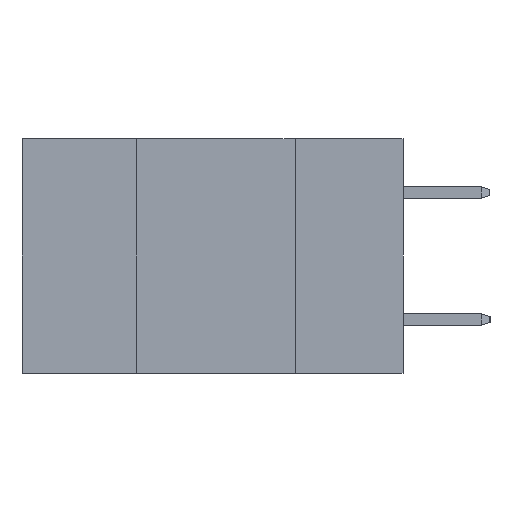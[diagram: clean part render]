
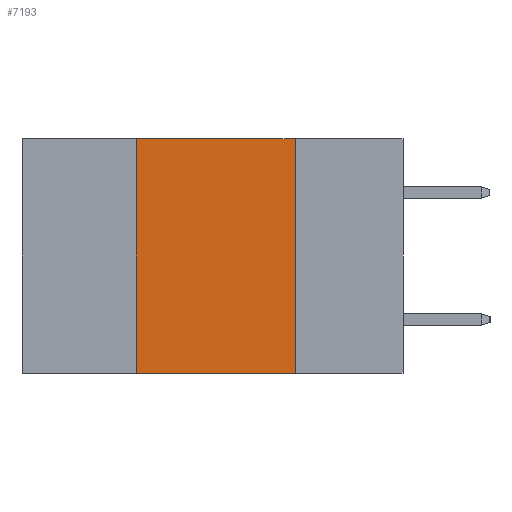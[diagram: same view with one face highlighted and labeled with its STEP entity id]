
A CAD part, left-side view. The second image highlights one B-rep face of the part: STEP entity #7193.
In plain terms, the highlighted planar face has unit normal (-1, 0, 0).
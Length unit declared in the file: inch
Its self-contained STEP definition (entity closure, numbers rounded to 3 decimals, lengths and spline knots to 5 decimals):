
#375 = CARTESIAN_POINT ( 'NONE',  ( 0., 0.42, 0. ) ) ;
#412 = CARTESIAN_POINT ( 'NONE',  ( 0., 0.6, 0. ) ) ;
#501 = EDGE_LOOP ( 'NONE', ( #10913, #5267, #13035, #7974 ) ) ;
#1068 = LINE ( 'NONE', #7234, #1835 ) ;
#1313 = CARTESIAN_POINT ( 'NONE',  ( 0., 0.42, 0. ) ) ;
#1835 = VECTOR ( 'NONE', #4190, 39.37008 ) ;
#2723 = VERTEX_POINT ( 'NONE', #14095 ) ;
#3085 = DIRECTION ( 'NONE',  ( 0., 0., -1. ) ) ;
#3303 = VERTEX_POINT ( 'NONE', #8169 ) ;
#3322 = VERTEX_POINT ( 'NONE', #375 ) ;
#4190 = DIRECTION ( 'NONE',  ( 0., 0., -1. ) ) ;
#4582 = LINE ( 'NONE', #5906, #6327 ) ;
#5114 = AXIS2_PLACEMENT_3D ( 'NONE', #10607, #6143, #3085 ) ;
#5267 = ORIENTED_EDGE ( 'NONE', *, *, #6508, .F. ) ;
#5906 = CARTESIAN_POINT ( 'NONE',  ( 0., 0.6, -0.37 ) ) ;
#6143 = DIRECTION ( 'NONE',  ( 1., 0., 0. ) ) ;
#6327 = VECTOR ( 'NONE', #15451, 39.37008 ) ;
#6508 = EDGE_CURVE ( 'NONE', #3322, #11072, #12897, .T. ) ;
#7193 = ADVANCED_FACE ( 'NONE', ( #19966 ), #18652, .F. ) ;
#7234 = CARTESIAN_POINT ( 'NONE',  ( 0., 0.17, 0. ) ) ;
#7974 = ORIENTED_EDGE ( 'NONE', *, *, #15948, .T. ) ;
#8125 = VECTOR ( 'NONE', #17045, 39.37008 ) ;
#8169 = CARTESIAN_POINT ( 'NONE',  ( 0., 0.17, -0.37 ) ) ;
#9642 = DIRECTION ( 'NONE',  ( 0., -1., 0. ) ) ;
#10607 = CARTESIAN_POINT ( 'NONE',  ( 0., 0.6, 0. ) ) ;
#10913 = ORIENTED_EDGE ( 'NONE', *, *, #19184, .F. ) ;
#11072 = VERTEX_POINT ( 'NONE', #16658 ) ;
#11674 = EDGE_CURVE ( 'NONE', #2723, #3322, #19893, .T. ) ;
#12897 = LINE ( 'NONE', #412, #13851 ) ;
#13035 = ORIENTED_EDGE ( 'NONE', *, *, #11674, .F. ) ;
#13851 = VECTOR ( 'NONE', #9642, 39.37008 ) ;
#14095 = CARTESIAN_POINT ( 'NONE',  ( 0., 0.42, -0.37 ) ) ;
#15451 = DIRECTION ( 'NONE',  ( 0., -1., 0. ) ) ;
#15948 = EDGE_CURVE ( 'NONE', #2723, #3303, #4582, .T. ) ;
#16658 = CARTESIAN_POINT ( 'NONE',  ( 0., 0.17, 0. ) ) ;
#17045 = DIRECTION ( 'NONE',  ( 0., 0., 1. ) ) ;
#18652 = PLANE ( 'NONE',  #5114 ) ;
#19184 = EDGE_CURVE ( 'NONE', #11072, #3303, #1068, .T. ) ;
#19893 = LINE ( 'NONE', #1313, #8125 ) ;
#19966 = FACE_OUTER_BOUND ( 'NONE', #501, .T. ) ;
